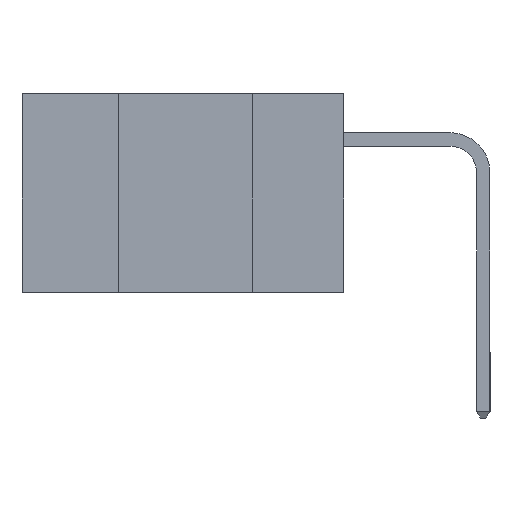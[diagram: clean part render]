
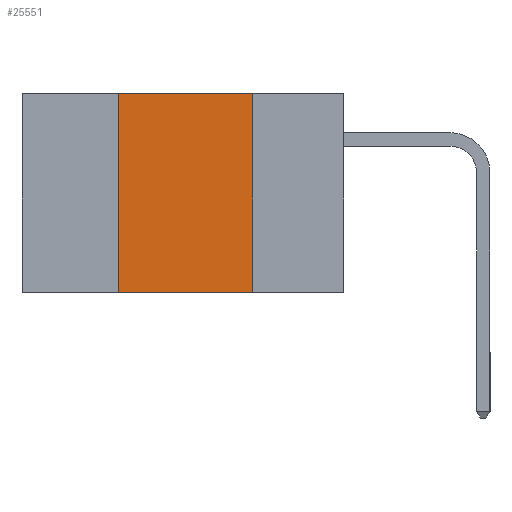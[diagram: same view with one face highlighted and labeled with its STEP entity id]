
A CAD part, left-side view. The second image highlights one B-rep face of the part: STEP entity #25551.
In plain terms, the highlighted planar face has unit normal (-1, 0, 0).
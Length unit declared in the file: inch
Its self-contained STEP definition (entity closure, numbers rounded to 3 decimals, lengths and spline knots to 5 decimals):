
#913 = EDGE_CURVE ( 'NONE', #3077, #11274, #1796, .T. ) ;
#1408 = CARTESIAN_POINT ( 'NONE',  ( 0., 0.17, -0.37 ) ) ;
#1796 = LINE ( 'NONE', #17341, #13963 ) ;
#2357 = DIRECTION ( 'NONE',  ( 0., 0., -1. ) ) ;
#2384 = EDGE_CURVE ( 'NONE', #10002, #18805, #27894, .T. ) ;
#3005 = LINE ( 'NONE', #8609, #6053 ) ;
#3030 = EDGE_CURVE ( 'NONE', #11274, #18805, #15351, .T. ) ;
#3077 = VERTEX_POINT ( 'NONE', #6258 ) ;
#3253 = ORIENTED_EDGE ( 'NONE', *, *, #13001, .F. ) ;
#3586 = CARTESIAN_POINT ( 'NONE',  ( 0., 0.17, 0. ) ) ;
#3602 = CARTESIAN_POINT ( 'NONE',  ( 0., 0.17, 0. ) ) ;
#4667 = EDGE_LOOP ( 'NONE', ( #27113, #7402, #3253, #14738 ) ) ;
#6039 = CARTESIAN_POINT ( 'NONE',  ( 0., 0.6, -0.37 ) ) ;
#6053 = VECTOR ( 'NONE', #11051, 39.37008 ) ;
#6100 = DIRECTION ( 'NONE',  ( 0., -1., 0. ) ) ;
#6258 = CARTESIAN_POINT ( 'NONE',  ( 0., 0.42, 0. ) ) ;
#7402 = ORIENTED_EDGE ( 'NONE', *, *, #913, .F. ) ;
#8446 = CARTESIAN_POINT ( 'NONE',  ( 0., 0.42, -0.37 ) ) ;
#8609 = CARTESIAN_POINT ( 'NONE',  ( 0., 0.42, 0. ) ) ;
#10002 = VERTEX_POINT ( 'NONE', #8446 ) ;
#10336 = DIRECTION ( 'NONE',  ( 0., -1., 0. ) ) ;
#11051 = DIRECTION ( 'NONE',  ( 0., 0., 1. ) ) ;
#11274 = VERTEX_POINT ( 'NONE', #3602 ) ;
#11708 = AXIS2_PLACEMENT_3D ( 'NONE', #31349, #16948, #2357 ) ;
#13001 = EDGE_CURVE ( 'NONE', #10002, #3077, #3005, .T. ) ;
#13357 = DIRECTION ( 'NONE',  ( 0., 0., -1. ) ) ;
#13963 = VECTOR ( 'NONE', #10336, 39.37008 ) ;
#14738 = ORIENTED_EDGE ( 'NONE', *, *, #2384, .T. ) ;
#15013 = VECTOR ( 'NONE', #6100, 39.37008 ) ;
#15351 = LINE ( 'NONE', #3586, #27477 ) ;
#16948 = DIRECTION ( 'NONE',  ( 1., 0., 0. ) ) ;
#16964 = FACE_OUTER_BOUND ( 'NONE', #4667, .T. ) ;
#17341 = CARTESIAN_POINT ( 'NONE',  ( 0., 0.6, 0. ) ) ;
#18805 = VERTEX_POINT ( 'NONE', #1408 ) ;
#25551 = ADVANCED_FACE ( 'NONE', ( #16964 ), #28974, .F. ) ;
#27113 = ORIENTED_EDGE ( 'NONE', *, *, #3030, .F. ) ;
#27477 = VECTOR ( 'NONE', #13357, 39.37008 ) ;
#27894 = LINE ( 'NONE', #6039, #15013 ) ;
#28974 = PLANE ( 'NONE',  #11708 ) ;
#31349 = CARTESIAN_POINT ( 'NONE',  ( 0., 0.6, 0. ) ) ;
